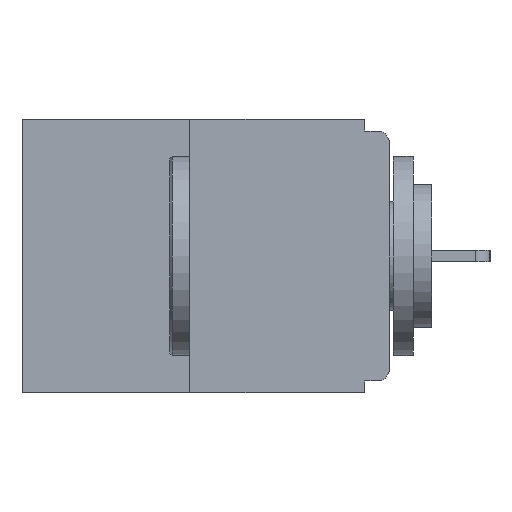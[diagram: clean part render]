
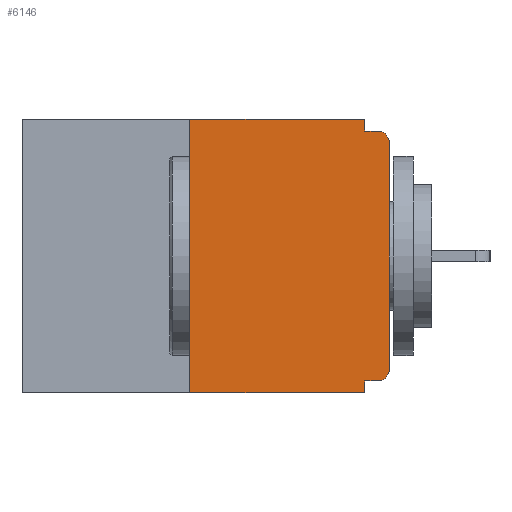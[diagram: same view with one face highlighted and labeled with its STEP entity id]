
A CAD part, left-side view. The second image highlights one B-rep face of the part: STEP entity #6146.
In plain terms, the highlighted planar face has unit normal (-1, 0, 0).
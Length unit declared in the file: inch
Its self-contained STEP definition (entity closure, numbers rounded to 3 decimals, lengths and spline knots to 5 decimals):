
#5 = VERTEX_POINT ( 'NONE', #10935 ) ;
#49 = LINE ( 'NONE', #5686, #2301 ) ;
#77 = CARTESIAN_POINT ( 'NONE',  ( 0., 0.25, 0. ) ) ;
#211 = LINE ( 'NONE', #7837, #7446 ) ;
#246 = ORIENTED_EDGE ( 'NONE', *, *, #12105, .T. ) ;
#261 = CARTESIAN_POINT ( 'NONE',  ( 0., 0.031, -0.015 ) ) ;
#750 = CARTESIAN_POINT ( 'NONE',  ( 0., 0.25, 0. ) ) ;
#1036 = AXIS2_PLACEMENT_3D ( 'NONE', #10059, #8855, #11128 ) ;
#1251 = LINE ( 'NONE', #77, #13930 ) ;
#1405 = DIRECTION ( 'NONE',  ( 0., -1., 0. ) ) ;
#1504 = CIRCLE ( 'NONE', #1036, 0.015 ) ;
#1737 = CARTESIAN_POINT ( 'NONE',  ( 0., 0.031, 0. ) ) ;
#2018 = EDGE_CURVE ( 'NONE', #8451, #11203, #5401, .T. ) ;
#2070 = CARTESIAN_POINT ( 'NONE',  ( 0., 0.015, -0.03 ) ) ;
#2130 = CARTESIAN_POINT ( 'NONE',  ( 0., 0.015, -0.015 ) ) ;
#2301 = VECTOR ( 'NONE', #10194, 39.37008 ) ;
#2438 = CARTESIAN_POINT ( 'NONE',  ( 0., 0.031, -0.343 ) ) ;
#2452 = ORIENTED_EDGE ( 'NONE', *, *, #3528, .T. ) ;
#2469 = CARTESIAN_POINT ( 'NONE',  ( 0., 0.015, -0.328 ) ) ;
#2475 = EDGE_CURVE ( 'NONE', #2756, #11203, #10259, .T. ) ;
#2545 = VERTEX_POINT ( 'NONE', #4319 ) ;
#2553 = CARTESIAN_POINT ( 'NONE',  ( 0., 0., -0.313 ) ) ;
#2756 = VERTEX_POINT ( 'NONE', #11129 ) ;
#2773 = EDGE_LOOP ( 'NONE', ( #4149, #13592, #246, #7395, #9837, #4659, #2452, #6406, #14140, #6891 ) ) ;
#3123 = CARTESIAN_POINT ( 'NONE',  ( 0., 0., -0.015 ) ) ;
#3326 = CARTESIAN_POINT ( 'NONE',  ( 0., 0.46, 0. ) ) ;
#3466 = VECTOR ( 'NONE', #8766, 39.37008 ) ;
#3528 = EDGE_CURVE ( 'NONE', #10793, #2756, #211, .T. ) ;
#3615 = EDGE_CURVE ( 'NONE', #5, #8451, #4015, .T. ) ;
#4012 = EDGE_CURVE ( 'NONE', #2545, #8821, #49, .T. ) ;
#4015 = LINE ( 'NONE', #1737, #9078 ) ;
#4149 = ORIENTED_EDGE ( 'NONE', *, *, #8882, .F. ) ;
#4319 = CARTESIAN_POINT ( 'NONE',  ( 0., 0.031, -0.328 ) ) ;
#4575 = VECTOR ( 'NONE', #13673, 39.37008 ) ;
#4659 = ORIENTED_EDGE ( 'NONE', *, *, #7060, .T. ) ;
#4715 = CARTESIAN_POINT ( 'NONE',  ( 0., 0.46, 0. ) ) ;
#5401 = LINE ( 'NONE', #3123, #3466 ) ;
#5686 = CARTESIAN_POINT ( 'NONE',  ( 0., 0.031, -0.343 ) ) ;
#5793 = DIRECTION ( 'NONE',  ( 0., 0., 1. ) ) ;
#6146 = ADVANCED_FACE ( 'NONE', ( #8901 ), #13378, .F. ) ;
#6351 = AXIS2_PLACEMENT_3D ( 'NONE', #3326, #7792, #12272 ) ;
#6406 = ORIENTED_EDGE ( 'NONE', *, *, #2475, .T. ) ;
#6891 = ORIENTED_EDGE ( 'NONE', *, *, #3615, .F. ) ;
#6908 = LINE ( 'NONE', #11472, #7198 ) ;
#7060 = EDGE_CURVE ( 'NONE', #12948, #10793, #1504, .T. ) ;
#7198 = VECTOR ( 'NONE', #1405, 39.37008 ) ;
#7395 = ORIENTED_EDGE ( 'NONE', *, *, #4012, .F. ) ;
#7446 = VECTOR ( 'NONE', #13495, 39.37008 ) ;
#7635 = VERTEX_POINT ( 'NONE', #750 ) ;
#7792 = DIRECTION ( 'NONE',  ( 1., 0., 0. ) ) ;
#7837 = CARTESIAN_POINT ( 'NONE',  ( 0., 0., 0. ) ) ;
#8018 = EDGE_CURVE ( 'NONE', #11002, #7635, #1251, .T. ) ;
#8451 = VERTEX_POINT ( 'NONE', #261 ) ;
#8766 = DIRECTION ( 'NONE',  ( 0., -1., 0. ) ) ;
#8821 = VERTEX_POINT ( 'NONE', #2438 ) ;
#8855 = DIRECTION ( 'NONE',  ( -1., 0., 0. ) ) ;
#8882 = EDGE_CURVE ( 'NONE', #7635, #5, #13746, .T. ) ;
#8901 = FACE_OUTER_BOUND ( 'NONE', #2773, .T. ) ;
#9078 = VECTOR ( 'NONE', #13856, 39.37008 ) ;
#9538 = AXIS2_PLACEMENT_3D ( 'NONE', #2070, #10002, #10152 ) ;
#9837 = ORIENTED_EDGE ( 'NONE', *, *, #11100, .F. ) ;
#10002 = DIRECTION ( 'NONE',  ( -1., 0., 0. ) ) ;
#10059 = CARTESIAN_POINT ( 'NONE',  ( 0., 0.015, -0.313 ) ) ;
#10152 = DIRECTION ( 'NONE',  ( 0., 0., -1. ) ) ;
#10194 = DIRECTION ( 'NONE',  ( 0., 0., -1. ) ) ;
#10259 = CIRCLE ( 'NONE', #9538, 0.015 ) ;
#10708 = VECTOR ( 'NONE', #11889, 39.37008 ) ;
#10793 = VERTEX_POINT ( 'NONE', #2553 ) ;
#10935 = CARTESIAN_POINT ( 'NONE',  ( 0., 0.031, 0. ) ) ;
#11002 = VERTEX_POINT ( 'NONE', #13872 ) ;
#11100 = EDGE_CURVE ( 'NONE', #12948, #2545, #13206, .T. ) ;
#11128 = DIRECTION ( 'NONE',  ( 0., 0., -1. ) ) ;
#11129 = CARTESIAN_POINT ( 'NONE',  ( 0., 0., -0.03 ) ) ;
#11203 = VERTEX_POINT ( 'NONE', #2130 ) ;
#11472 = CARTESIAN_POINT ( 'NONE',  ( 0., 0.46, -0.343 ) ) ;
#11889 = DIRECTION ( 'NONE',  ( 0., 1., 0. ) ) ;
#12105 = EDGE_CURVE ( 'NONE', #11002, #8821, #6908, .T. ) ;
#12272 = DIRECTION ( 'NONE',  ( 0., 0., -1. ) ) ;
#12948 = VERTEX_POINT ( 'NONE', #2469 ) ;
#13206 = LINE ( 'NONE', #14082, #10708 ) ;
#13378 = PLANE ( 'NONE',  #6351 ) ;
#13495 = DIRECTION ( 'NONE',  ( 0., 0., 1. ) ) ;
#13592 = ORIENTED_EDGE ( 'NONE', *, *, #8018, .F. ) ;
#13673 = DIRECTION ( 'NONE',  ( 0., -1., 0. ) ) ;
#13746 = LINE ( 'NONE', #4715, #4575 ) ;
#13856 = DIRECTION ( 'NONE',  ( 0., 0., -1. ) ) ;
#13872 = CARTESIAN_POINT ( 'NONE',  ( 0., 0.25, -0.343 ) ) ;
#13930 = VECTOR ( 'NONE', #5793, 39.37008 ) ;
#14082 = CARTESIAN_POINT ( 'NONE',  ( 0., 0., -0.328 ) ) ;
#14140 = ORIENTED_EDGE ( 'NONE', *, *, #2018, .F. ) ;
